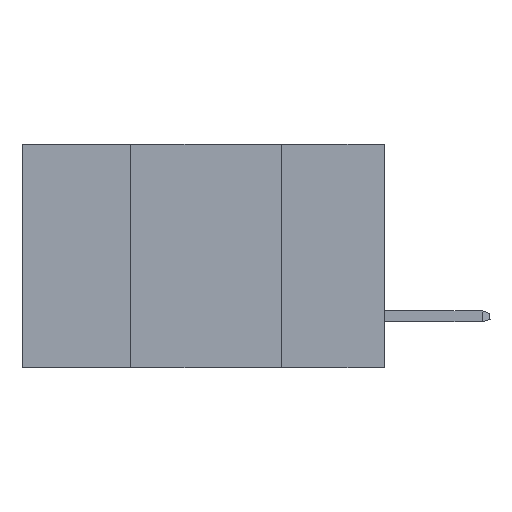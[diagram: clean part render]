
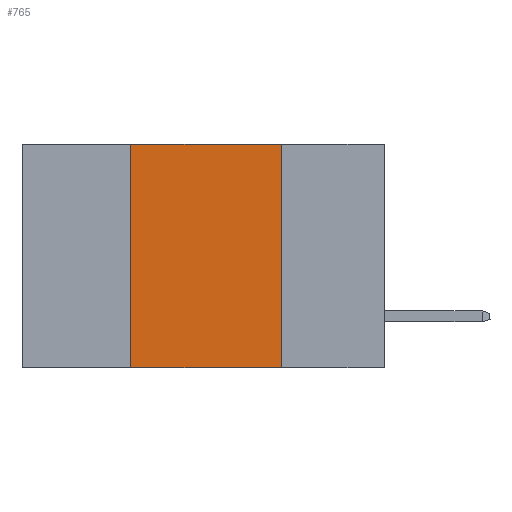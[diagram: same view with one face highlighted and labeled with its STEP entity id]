
A CAD part, left-side view. The second image highlights one B-rep face of the part: STEP entity #765.
In plain terms, the highlighted planar face has unit normal (-1, 0, 0).
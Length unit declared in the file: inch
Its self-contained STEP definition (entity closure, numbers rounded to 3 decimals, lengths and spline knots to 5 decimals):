
#289 = CARTESIAN_POINT ( 'NONE',  ( 0., 0.17, -0.37 ) ) ;
#765 = ADVANCED_FACE ( 'NONE', ( #7270 ), #7653, .F. ) ;
#934 = CARTESIAN_POINT ( 'NONE',  ( 0., 0.42, -0.37 ) ) ;
#973 = CARTESIAN_POINT ( 'NONE',  ( 0., 0.6, 0. ) ) ;
#1073 = ORIENTED_EDGE ( 'NONE', *, *, #3025, .T. ) ;
#1319 = DIRECTION ( 'NONE',  ( 0., 0., -1. ) ) ;
#1748 = VECTOR ( 'NONE', #4046, 39.37008 ) ;
#1891 = LINE ( 'NONE', #4290, #2547 ) ;
#1941 = AXIS2_PLACEMENT_3D ( 'NONE', #10815, #10860, #6758 ) ;
#2547 = VECTOR ( 'NONE', #7447, 39.37008 ) ;
#2975 = DIRECTION ( 'NONE',  ( 0., -1., 0. ) ) ;
#3025 = EDGE_CURVE ( 'NONE', #8792, #10490, #4554, .T. ) ;
#3804 = VECTOR ( 'NONE', #1319, 39.37008 ) ;
#4046 = DIRECTION ( 'NONE',  ( 0., -1., 0. ) ) ;
#4290 = CARTESIAN_POINT ( 'NONE',  ( 0., 0.42, -0.37 ) ) ;
#4554 = LINE ( 'NONE', #12550, #1748 ) ;
#4840 = CARTESIAN_POINT ( 'NONE',  ( 0., 0.17, 0. ) ) ;
#5230 = VERTEX_POINT ( 'NONE', #8391 ) ;
#5696 = EDGE_CURVE ( 'NONE', #5230, #11706, #12138, .T. ) ;
#6032 = EDGE_LOOP ( 'NONE', ( #8610, #10199, #7004, #1073 ) ) ;
#6758 = DIRECTION ( 'NONE',  ( 0., 0., -1. ) ) ;
#6828 = EDGE_CURVE ( 'NONE', #11706, #10490, #10956, .T. ) ;
#7004 = ORIENTED_EDGE ( 'NONE', *, *, #13766, .F. ) ;
#7264 = VECTOR ( 'NONE', #2975, 39.37008 ) ;
#7270 = FACE_OUTER_BOUND ( 'NONE', #6032, .T. ) ;
#7447 = DIRECTION ( 'NONE',  ( 0., 0., 1. ) ) ;
#7653 = PLANE ( 'NONE',  #1941 ) ;
#8391 = CARTESIAN_POINT ( 'NONE',  ( 0., 0.42, 0. ) ) ;
#8610 = ORIENTED_EDGE ( 'NONE', *, *, #6828, .F. ) ;
#8792 = VERTEX_POINT ( 'NONE', #934 ) ;
#10199 = ORIENTED_EDGE ( 'NONE', *, *, #5696, .F. ) ;
#10490 = VERTEX_POINT ( 'NONE', #12588 ) ;
#10815 = CARTESIAN_POINT ( 'NONE',  ( 0., 0.6, 0. ) ) ;
#10860 = DIRECTION ( 'NONE',  ( 1., 0., 0. ) ) ;
#10956 = LINE ( 'NONE', #289, #3804 ) ;
#11706 = VERTEX_POINT ( 'NONE', #4840 ) ;
#12138 = LINE ( 'NONE', #973, #7264 ) ;
#12550 = CARTESIAN_POINT ( 'NONE',  ( 0., 0.6, -0.37 ) ) ;
#12588 = CARTESIAN_POINT ( 'NONE',  ( 0., 0.17, -0.37 ) ) ;
#13766 = EDGE_CURVE ( 'NONE', #8792, #5230, #1891, .T. ) ;
